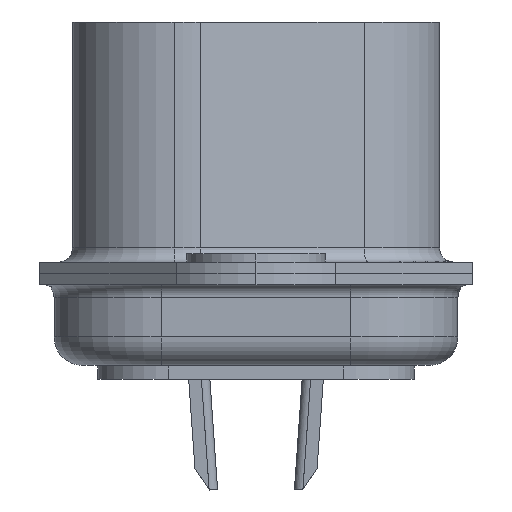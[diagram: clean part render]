
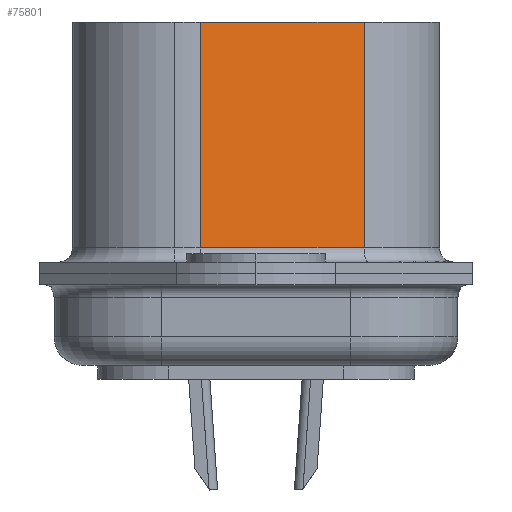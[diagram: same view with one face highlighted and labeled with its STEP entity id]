
A CAD part, left-side view. The second image highlights one B-rep face of the part: STEP entity #75801.
In plain terms, the highlighted planar face has unit normal (-0.966, -0.259, 0).
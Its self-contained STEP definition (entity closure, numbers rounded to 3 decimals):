
#10137 = ORIENTED_EDGE ( 'NONE', *, *, #18074, .F. ) ;
#13940 = DIRECTION ( 'NONE',  ( 0.259, -0.966, 0. ) ) ;
#18074 = EDGE_CURVE ( 'NONE', #138993, #81893, #62805, .T. ) ;
#28430 = CARTESIAN_POINT ( 'NONE',  ( 4.913, 1.968, 9.3 ) ) ;
#32734 = ORIENTED_EDGE ( 'NONE', *, *, #109426, .T. ) ;
#40333 = LINE ( 'NONE', #28430, #165019 ) ;
#40769 = VECTOR ( 'NONE', #52552, 1000. ) ;
#46886 = EDGE_CURVE ( 'NONE', #99750, #138993, #103119, .T. ) ;
#51321 = VECTOR ( 'NONE', #13940, 1000. ) ;
#52552 = DIRECTION ( 'NONE',  ( 0., 0., -1. ) ) ;
#53677 = CARTESIAN_POINT ( 'NONE',  ( 6.467, -3.832, 1.3 ) ) ;
#54616 = CARTESIAN_POINT ( 'NONE',  ( 6.467, -3.832, 9.3 ) ) ;
#61145 = ORIENTED_EDGE ( 'NONE', *, *, #93893, .T. ) ;
#62805 = LINE ( 'NONE', #139998, #40769 ) ;
#64522 = FACE_OUTER_BOUND ( 'NONE', #133838, .T. ) ;
#75801 = ADVANCED_FACE ( 'NONE', ( #64522 ), #90821, .F. ) ;
#78739 = AXIS2_PLACEMENT_3D ( 'NONE', #142517, #167156, #154426 ) ;
#79266 = VECTOR ( 'NONE', #100586, 1000. ) ;
#80194 = DIRECTION ( 'NONE',  ( 0., 0., -1. ) ) ;
#81893 = VERTEX_POINT ( 'NONE', #53677 ) ;
#90821 = PLANE ( 'NONE',  #78739 ) ;
#93893 = EDGE_CURVE ( 'NONE', #99750, #134230, #40333, .T. ) ;
#97683 = CARTESIAN_POINT ( 'NONE',  ( 4.913, 1.968, 1.3 ) ) ;
#99750 = VERTEX_POINT ( 'NONE', #149727 ) ;
#100586 = DIRECTION ( 'NONE',  ( 0.259, -0.966, 0. ) ) ;
#103119 = LINE ( 'NONE', #54616, #51321 ) ;
#109426 = EDGE_CURVE ( 'NONE', #134230, #81893, #152292, .T. ) ;
#111541 = CARTESIAN_POINT ( 'NONE',  ( 6.467, -3.832, 9.3 ) ) ;
#112483 = CARTESIAN_POINT ( 'NONE',  ( 6.467, -3.832, 1.3 ) ) ;
#133838 = EDGE_LOOP ( 'NONE', ( #61145, #32734, #10137, #164300 ) ) ;
#134230 = VERTEX_POINT ( 'NONE', #97683 ) ;
#138993 = VERTEX_POINT ( 'NONE', #111541 ) ;
#139998 = CARTESIAN_POINT ( 'NONE',  ( 6.467, -3.832, 9.3 ) ) ;
#142517 = CARTESIAN_POINT ( 'NONE',  ( 6.467, -3.832, 9.3 ) ) ;
#149727 = CARTESIAN_POINT ( 'NONE',  ( 4.913, 1.968, 9.3 ) ) ;
#152292 = LINE ( 'NONE', #112483, #79266 ) ;
#154426 = DIRECTION ( 'NONE',  ( -0.259, 0.966, 0. ) ) ;
#164300 = ORIENTED_EDGE ( 'NONE', *, *, #46886, .F. ) ;
#165019 = VECTOR ( 'NONE', #80194, 1000. ) ;
#167156 = DIRECTION ( 'NONE',  ( 0.966, 0.259, 0. ) ) ;
